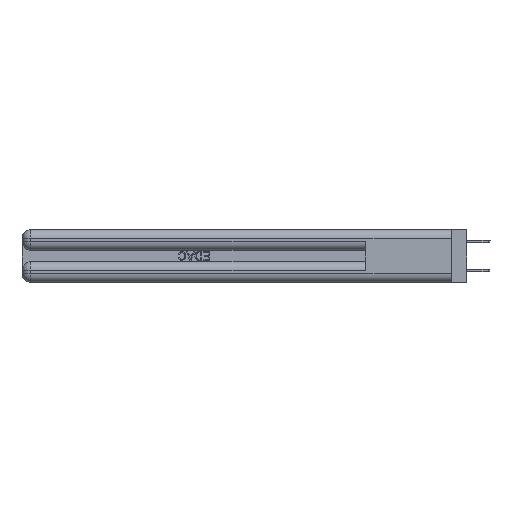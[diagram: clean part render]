
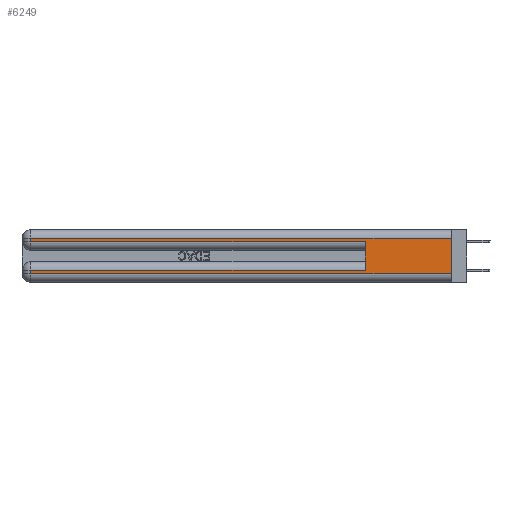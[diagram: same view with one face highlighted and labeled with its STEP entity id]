
A CAD part, left-side view. The second image highlights one B-rep face of the part: STEP entity #6249.
In plain terms, the highlighted planar face has unit normal (-1, 0, 0).
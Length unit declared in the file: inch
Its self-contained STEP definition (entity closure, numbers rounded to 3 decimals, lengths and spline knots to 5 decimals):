
#548 = VECTOR ( 'NONE', #33551, 39.37008 ) ;
#1183 = VECTOR ( 'NONE', #11820, 39.37008 ) ;
#1233 = EDGE_CURVE ( 'NONE', #17974, #28576, #4441, .T. ) ;
#2349 = LINE ( 'NONE', #18964, #40716 ) ;
#3015 = VERTEX_POINT ( 'NONE', #25981 ) ;
#3378 = LINE ( 'NONE', #38110, #32430 ) ;
#4441 = LINE ( 'NONE', #35714, #42838 ) ;
#4514 = VERTEX_POINT ( 'NONE', #23406 ) ;
#6249 = ADVANCED_FACE ( 'NONE', ( #17071 ), #37635, .F. ) ;
#7541 = CARTESIAN_POINT ( 'NONE',  ( 0., 0., 0.06 ) ) ;
#8189 = CARTESIAN_POINT ( 'NONE',  ( 0., 0.6, 0.085 ) ) ;
#8466 = VECTOR ( 'NONE', #47775, 39.37008 ) ;
#9265 = ORIENTED_EDGE ( 'NONE', *, *, #42737, .T. ) ;
#10457 = DIRECTION ( 'NONE',  ( 0., 0., -1. ) ) ;
#11421 = VERTEX_POINT ( 'NONE', #42425 ) ;
#11820 = DIRECTION ( 'NONE',  ( 0., 1., 0. ) ) ;
#14526 = EDGE_CURVE ( 'NONE', #4514, #11421, #44489, .T. ) ;
#15995 = DIRECTION ( 'NONE',  ( 0., -1., 0. ) ) ;
#16016 = ORIENTED_EDGE ( 'NONE', *, *, #25194, .T. ) ;
#16163 = DIRECTION ( 'NONE',  ( 1., 0., 0. ) ) ;
#16564 = ORIENTED_EDGE ( 'NONE', *, *, #17704, .T. ) ;
#17071 = FACE_OUTER_BOUND ( 'NONE', #33846, .T. ) ;
#17704 = EDGE_CURVE ( 'NONE', #11421, #18241, #35819, .T. ) ;
#17974 = VERTEX_POINT ( 'NONE', #34525 ) ;
#18227 = CARTESIAN_POINT ( 'NONE',  ( 0., 2.94, 0.285 ) ) ;
#18241 = VERTEX_POINT ( 'NONE', #7541 ) ;
#18760 = ORIENTED_EDGE ( 'NONE', *, *, #29968, .F. ) ;
#18964 = CARTESIAN_POINT ( 'NONE',  ( 0., 0., 0.085 ) ) ;
#19821 = LINE ( 'NONE', #40478, #1183 ) ;
#19892 = ORIENTED_EDGE ( 'NONE', *, *, #14526, .T. ) ;
#21289 = CARTESIAN_POINT ( 'NONE',  ( 0., 2.94, 0.37 ) ) ;
#22750 = VERTEX_POINT ( 'NONE', #8189 ) ;
#23406 = CARTESIAN_POINT ( 'NONE',  ( 0., 2.94, 0.085 ) ) ;
#24298 = ORIENTED_EDGE ( 'NONE', *, *, #38731, .F. ) ;
#24948 = ORIENTED_EDGE ( 'NONE', *, *, #1233, .T. ) ;
#25194 = EDGE_CURVE ( 'NONE', #28576, #26811, #3378, .T. ) ;
#25981 = CARTESIAN_POINT ( 'NONE',  ( 0., 0., 0.31 ) ) ;
#26458 = DIRECTION ( 'NONE',  ( 0., 1., 0. ) ) ;
#26811 = VERTEX_POINT ( 'NONE', #27767 ) ;
#27450 = DIRECTION ( 'NONE',  ( 0., -1., 0. ) ) ;
#27767 = CARTESIAN_POINT ( 'NONE',  ( 0., 0.6, 0.285 ) ) ;
#28576 = VERTEX_POINT ( 'NONE', #18227 ) ;
#29072 = EDGE_CURVE ( 'NONE', #3015, #17974, #19821, .T. ) ;
#29646 = LINE ( 'NONE', #33869, #548 ) ;
#29968 = EDGE_CURVE ( 'NONE', #22750, #26811, #29646, .T. ) ;
#31151 = AXIS2_PLACEMENT_3D ( 'NONE', #47337, #16163, #10457 ) ;
#32332 = LINE ( 'NONE', #40760, #8466 ) ;
#32430 = VECTOR ( 'NONE', #15995, 39.37008 ) ;
#33551 = DIRECTION ( 'NONE',  ( 0., 0., 1. ) ) ;
#33846 = EDGE_LOOP ( 'NONE', ( #24298, #36522, #24948, #16016, #18760, #9265, #19892, #16564 ) ) ;
#33869 = CARTESIAN_POINT ( 'NONE',  ( 0., 0.6, 0.145 ) ) ;
#33966 = VECTOR ( 'NONE', #36213, 39.37008 ) ;
#34525 = CARTESIAN_POINT ( 'NONE',  ( 0., 2.94, 0.31 ) ) ;
#35714 = CARTESIAN_POINT ( 'NONE',  ( 0., 2.94, 0.37 ) ) ;
#35819 = LINE ( 'NONE', #38452, #37520 ) ;
#36213 = DIRECTION ( 'NONE',  ( 0., 0., -1. ) ) ;
#36522 = ORIENTED_EDGE ( 'NONE', *, *, #29072, .T. ) ;
#37520 = VECTOR ( 'NONE', #27450, 39.37008 ) ;
#37635 = PLANE ( 'NONE',  #31151 ) ;
#38110 = CARTESIAN_POINT ( 'NONE',  ( 0., 0., 0.285 ) ) ;
#38452 = CARTESIAN_POINT ( 'NONE',  ( 0., 0., 0.06 ) ) ;
#38731 = EDGE_CURVE ( 'NONE', #3015, #18241, #32332, .T. ) ;
#40478 = CARTESIAN_POINT ( 'NONE',  ( 0., 0., 0.31 ) ) ;
#40716 = VECTOR ( 'NONE', #26458, 39.37008 ) ;
#40760 = CARTESIAN_POINT ( 'NONE',  ( 0., 0., 0.37 ) ) ;
#42425 = CARTESIAN_POINT ( 'NONE',  ( 0., 2.94, 0.06 ) ) ;
#42737 = EDGE_CURVE ( 'NONE', #22750, #4514, #2349, .T. ) ;
#42838 = VECTOR ( 'NONE', #46939, 39.37008 ) ;
#44489 = LINE ( 'NONE', #21289, #33966 ) ;
#46939 = DIRECTION ( 'NONE',  ( 0., 0., -1. ) ) ;
#47337 = CARTESIAN_POINT ( 'NONE',  ( 0., 0., 0.37 ) ) ;
#47775 = DIRECTION ( 'NONE',  ( 0., 0., -1. ) ) ;
